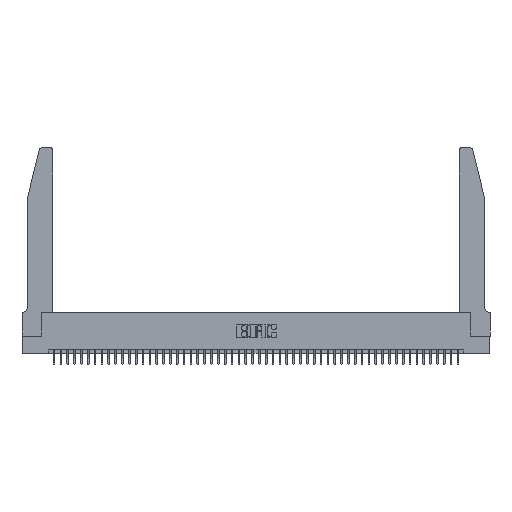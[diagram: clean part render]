
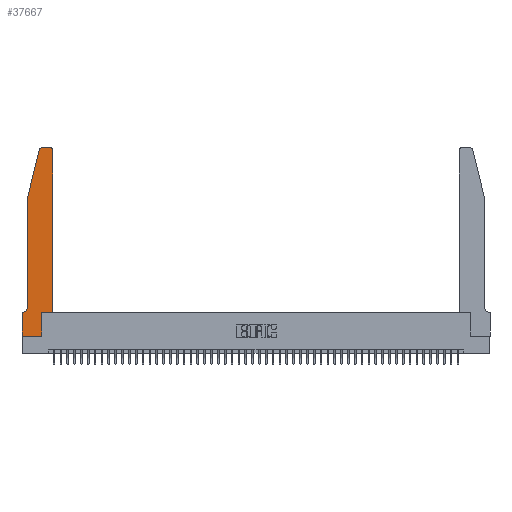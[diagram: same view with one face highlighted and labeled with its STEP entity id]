
A CAD part, top view. The second image highlights one B-rep face of the part: STEP entity #37667.
In plain terms, the highlighted planar face has unit normal (0, 0, 1).
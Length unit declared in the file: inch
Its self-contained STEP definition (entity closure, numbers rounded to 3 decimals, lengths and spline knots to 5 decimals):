
#544 = CARTESIAN_POINT ( 'NONE',  ( 0.0755, 0.35, 0.37 ) ) ;
#686 = DIRECTION ( 'NONE',  ( 0., 0., -1. ) ) ;
#1110 = EDGE_CURVE ( 'NONE', #1258, #3852, #4575, .T. ) ;
#1258 = VERTEX_POINT ( 'NONE', #37060 ) ;
#2015 = LINE ( 'NONE', #20528, #3182 ) ;
#2971 = VECTOR ( 'NONE', #16667, 39.37008 ) ;
#3182 = VECTOR ( 'NONE', #9116, 39.37008 ) ;
#3276 = DIRECTION ( 'NONE',  ( -1., 0., 0. ) ) ;
#3852 = VERTEX_POINT ( 'NONE', #10193 ) ;
#4575 = LINE ( 'NONE', #14464, #48340 ) ;
#4698 = EDGE_CURVE ( 'NONE', #20525, #17307, #46158, .T. ) ;
#6419 = VERTEX_POINT ( 'NONE', #29625 ) ;
#6688 = ORIENTED_EDGE ( 'NONE', *, *, #34827, .T. ) ;
#8715 = EDGE_CURVE ( 'NONE', #45876, #41771, #19580, .T. ) ;
#8827 = DIRECTION ( 'NONE',  ( 0., 1., 0. ) ) ;
#8942 = CARTESIAN_POINT ( 'NONE',  ( 0.4205, 2.75, 0.37 ) ) ;
#9116 = DIRECTION ( 'NONE',  ( -0.239, -0.971, 0. ) ) ;
#9148 = CARTESIAN_POINT ( 'NONE',  ( 0.0755, 2., 0.37 ) ) ;
#9209 = ORIENTED_EDGE ( 'NONE', *, *, #42787, .T. ) ;
#9467 = ORIENTED_EDGE ( 'NONE', *, *, #4698, .T. ) ;
#9538 = CIRCLE ( 'NONE', #40815, 0.03 ) ;
#9711 = ORIENTED_EDGE ( 'NONE', *, *, #40287, .T. ) ;
#10193 = CARTESIAN_POINT ( 'NONE',  ( 0.2865, 0., 0.37 ) ) ;
#10488 = CARTESIAN_POINT ( 'NONE',  ( 0.2865, 0.35, 0.37 ) ) ;
#11438 = DIRECTION ( 'NONE',  ( 1., 0., 0. ) ) ;
#11953 = LINE ( 'NONE', #26831, #31231 ) ;
#12359 = LINE ( 'NONE', #24091, #40564 ) ;
#13468 = EDGE_CURVE ( 'NONE', #42761, #45876, #30606, .T. ) ;
#13512 = ORIENTED_EDGE ( 'NONE', *, *, #41819, .T. ) ;
#13545 = ORIENTED_EDGE ( 'NONE', *, *, #27295, .T. ) ;
#14206 = VECTOR ( 'NONE', #42021, 39.37008 ) ;
#14464 = CARTESIAN_POINT ( 'NONE',  ( 0., 0., 0.37 ) ) ;
#14890 = CARTESIAN_POINT ( 'NONE',  ( 0.0055, 0.35, 0.37 ) ) ;
#16077 = EDGE_CURVE ( 'NONE', #39797, #6419, #12359, .T. ) ;
#16667 = DIRECTION ( 'NONE',  ( 0., -1., 0. ) ) ;
#16684 = CARTESIAN_POINT ( 'NONE',  ( 0.2865, 0.35, 0.37 ) ) ;
#16701 = CARTESIAN_POINT ( 'NONE',  ( 0., 0.35, 0.37 ) ) ;
#17065 = CARTESIAN_POINT ( 'NONE',  ( 0.25487, 2.72718, 0.37 ) ) ;
#17307 = VERTEX_POINT ( 'NONE', #28692 ) ;
#17475 = AXIS2_PLACEMENT_3D ( 'NONE', #16701, #32198, #43044 ) ;
#18183 = DIRECTION ( 'NONE',  ( 1., 0., 0. ) ) ;
#18388 = ORIENTED_EDGE ( 'NONE', *, *, #13468, .T. ) ;
#18903 = CARTESIAN_POINT ( 'NONE',  ( 0.4505, 0.35, 0.37 ) ) ;
#18975 = DIRECTION ( 'NONE',  ( -1., 0., 0. ) ) ;
#19580 = CIRCLE ( 'NONE', #29758, 0.07 ) ;
#19895 = CIRCLE ( 'NONE', #32364, 0.03 ) ;
#19932 = DIRECTION ( 'NONE',  ( -1., 0., 0. ) ) ;
#20525 = VERTEX_POINT ( 'NONE', #8942 ) ;
#20528 = CARTESIAN_POINT ( 'NONE',  ( 0.0755, 2., 0.37 ) ) ;
#20669 = ORIENTED_EDGE ( 'NONE', *, *, #24976, .T. ) ;
#21339 = VECTOR ( 'NONE', #18975, 39.37008 ) ;
#21923 = LINE ( 'NONE', #544, #21339 ) ;
#23116 = CARTESIAN_POINT ( 'NONE',  ( 0.4505, 2.72, 0.37 ) ) ;
#23336 = VERTEX_POINT ( 'NONE', #17065 ) ;
#23654 = EDGE_CURVE ( 'NONE', #6419, #42431, #24458, .T. ) ;
#24091 = CARTESIAN_POINT ( 'NONE',  ( 0.4505, 0.35, 0.37 ) ) ;
#24458 = LINE ( 'NONE', #18903, #14206 ) ;
#24924 = FACE_OUTER_BOUND ( 'NONE', #32074, .T. ) ;
#24959 = CARTESIAN_POINT ( 'NONE',  ( 0., 0.35, 0.37 ) ) ;
#24976 = EDGE_CURVE ( 'NONE', #41771, #39681, #21923, .T. ) ;
#25026 = ORIENTED_EDGE ( 'NONE', *, *, #8715, .T. ) ;
#26066 = ORIENTED_EDGE ( 'NONE', *, *, #23654, .T. ) ;
#26831 = CARTESIAN_POINT ( 'NONE',  ( 0., 0., 0.37 ) ) ;
#27295 = EDGE_CURVE ( 'NONE', #17307, #23336, #19895, .T. ) ;
#28692 = CARTESIAN_POINT ( 'NONE',  ( 0.284, 2.75, 0.37 ) ) ;
#28912 = ORIENTED_EDGE ( 'NONE', *, *, #16077, .T. ) ;
#29070 = ORIENTED_EDGE ( 'NONE', *, *, #1110, .T. ) ;
#29625 = CARTESIAN_POINT ( 'NONE',  ( 0.4505, 0.35, 0.37 ) ) ;
#29758 = AXIS2_PLACEMENT_3D ( 'NONE', #43229, #686, #19932 ) ;
#29918 = CARTESIAN_POINT ( 'NONE',  ( 0.0755, 0.42, 0.37 ) ) ;
#30606 = LINE ( 'NONE', #47387, #2971 ) ;
#30622 = CARTESIAN_POINT ( 'NONE',  ( 0.284, 2.72, 0.37 ) ) ;
#31231 = VECTOR ( 'NONE', #37733, 39.37008 ) ;
#31692 = PLANE ( 'NONE',  #17475 ) ;
#32074 = EDGE_LOOP ( 'NONE', ( #9467, #13545, #9711, #18388, #25026, #20669, #13512, #29070, #9209, #28912, #26066, #6688 ) ) ;
#32198 = DIRECTION ( 'NONE',  ( 0., 0., 1. ) ) ;
#32364 = AXIS2_PLACEMENT_3D ( 'NONE', #30622, #34492, #11438 ) ;
#32386 = VECTOR ( 'NONE', #3276, 39.37008 ) ;
#32885 = DIRECTION ( 'NONE',  ( 1., 0., 0. ) ) ;
#32917 = VECTOR ( 'NONE', #8827, 39.37008 ) ;
#34307 = CARTESIAN_POINT ( 'NONE',  ( 0.2605, 2.75, 0.37 ) ) ;
#34492 = DIRECTION ( 'NONE',  ( 0., 0., 1. ) ) ;
#34827 = EDGE_CURVE ( 'NONE', #42431, #20525, #9538, .T. ) ;
#37043 = DIRECTION ( 'NONE',  ( 0., 0., 1. ) ) ;
#37060 = CARTESIAN_POINT ( 'NONE',  ( 0., 0., 0.37 ) ) ;
#37667 = ADVANCED_FACE ( 'NONE', ( #24924 ), #31692, .T. ) ;
#37733 = DIRECTION ( 'NONE',  ( 0., -1., 0. ) ) ;
#39681 = VERTEX_POINT ( 'NONE', #24959 ) ;
#39797 = VERTEX_POINT ( 'NONE', #10488 ) ;
#40287 = EDGE_CURVE ( 'NONE', #23336, #42761, #2015, .T. ) ;
#40564 = VECTOR ( 'NONE', #47553, 39.37008 ) ;
#40815 = AXIS2_PLACEMENT_3D ( 'NONE', #47958, #37043, #32885 ) ;
#41771 = VERTEX_POINT ( 'NONE', #14890 ) ;
#41819 = EDGE_CURVE ( 'NONE', #39681, #1258, #11953, .T. ) ;
#42021 = DIRECTION ( 'NONE',  ( 0., 1., 0. ) ) ;
#42431 = VERTEX_POINT ( 'NONE', #23116 ) ;
#42761 = VERTEX_POINT ( 'NONE', #9148 ) ;
#42787 = EDGE_CURVE ( 'NONE', #3852, #39797, #43058, .T. ) ;
#43044 = DIRECTION ( 'NONE',  ( 1., 0., 0. ) ) ;
#43058 = LINE ( 'NONE', #16684, #32917 ) ;
#43229 = CARTESIAN_POINT ( 'NONE',  ( 0.0055, 0.42, 0.37 ) ) ;
#45876 = VERTEX_POINT ( 'NONE', #29918 ) ;
#46158 = LINE ( 'NONE', #34307, #32386 ) ;
#47387 = CARTESIAN_POINT ( 'NONE',  ( 0.0755, 2., 0.37 ) ) ;
#47553 = DIRECTION ( 'NONE',  ( 1., 0., 0. ) ) ;
#47958 = CARTESIAN_POINT ( 'NONE',  ( 0.4205, 2.72, 0.37 ) ) ;
#48340 = VECTOR ( 'NONE', #18183, 39.37008 ) ;
